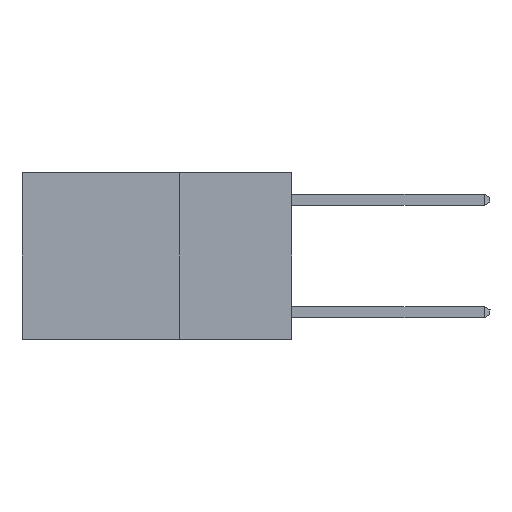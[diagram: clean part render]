
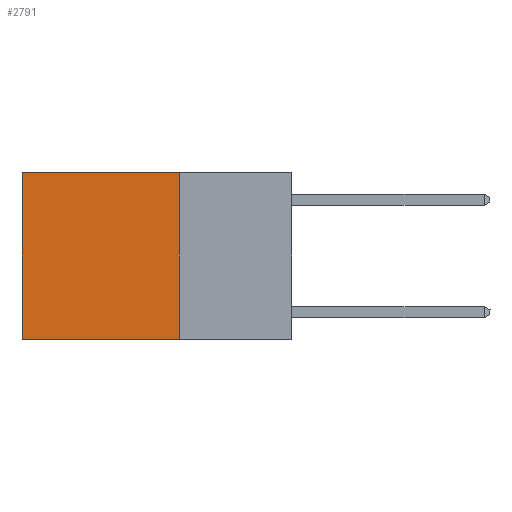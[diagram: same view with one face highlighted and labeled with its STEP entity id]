
A CAD part, left-side view. The second image highlights one B-rep face of the part: STEP entity #2791.
In plain terms, the highlighted planar face has unit normal (-1, 0, 0).
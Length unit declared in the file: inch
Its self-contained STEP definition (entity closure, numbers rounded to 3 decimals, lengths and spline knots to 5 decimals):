
#106 = CARTESIAN_POINT ( 'NONE',  ( 0.2625, 0.6, -0.37 ) ) ;
#130 = ORIENTED_EDGE ( 'NONE', *, *, #4910, .T. ) ;
#237 = ORIENTED_EDGE ( 'NONE', *, *, #2673, .T. ) ;
#852 = ORIENTED_EDGE ( 'NONE', *, *, #1747, .F. ) ;
#915 = ORIENTED_EDGE ( 'NONE', *, *, #6691, .F. ) ;
#1747 = EDGE_CURVE ( 'NONE', #3632, #5428, #7974, .T. ) ;
#1890 = LINE ( 'NONE', #3417, #10299 ) ;
#2107 = DIRECTION ( 'NONE',  ( 0., 1., 0. ) ) ;
#2298 = CARTESIAN_POINT ( 'NONE',  ( 0.2625, 0.25, 0. ) ) ;
#2512 = CARTESIAN_POINT ( 'NONE',  ( 0.2625, 0.6, 0. ) ) ;
#2673 = EDGE_CURVE ( 'NONE', #3632, #8798, #5055, .T. ) ;
#2791 = ADVANCED_FACE ( 'NONE', ( #6189 ), #8386, .F. ) ;
#2939 = VERTEX_POINT ( 'NONE', #106 ) ;
#2976 = CARTESIAN_POINT ( 'NONE',  ( 0.2625, 0.25, 0. ) ) ;
#3417 = CARTESIAN_POINT ( 'NONE',  ( 0.2625, 0.6, 0. ) ) ;
#3632 = VERTEX_POINT ( 'NONE', #2976 ) ;
#4337 = CARTESIAN_POINT ( 'NONE',  ( 0.2625, 0.25, 0. ) ) ;
#4779 = DIRECTION ( 'NONE',  ( 0., 0., -1. ) ) ;
#4910 = EDGE_CURVE ( 'NONE', #8798, #2939, #1890, .T. ) ;
#5055 = LINE ( 'NONE', #9016, #9066 ) ;
#5203 = DIRECTION ( 'NONE',  ( 0., 0., -1. ) ) ;
#5428 = VERTEX_POINT ( 'NONE', #7160 ) ;
#6189 = FACE_OUTER_BOUND ( 'NONE', #7083, .T. ) ;
#6691 = EDGE_CURVE ( 'NONE', #5428, #2939, #7344, .T. ) ;
#7083 = EDGE_LOOP ( 'NONE', ( #130, #915, #852, #237 ) ) ;
#7160 = CARTESIAN_POINT ( 'NONE',  ( 0.2625, 0.25, -0.37 ) ) ;
#7344 = LINE ( 'NONE', #7818, #9224 ) ;
#7622 = AXIS2_PLACEMENT_3D ( 'NONE', #4337, #9985, #5203 ) ;
#7818 = CARTESIAN_POINT ( 'NONE',  ( 0.2625, 0.25, -0.37 ) ) ;
#7974 = LINE ( 'NONE', #2298, #9844 ) ;
#8386 = PLANE ( 'NONE',  #7622 ) ;
#8798 = VERTEX_POINT ( 'NONE', #2512 ) ;
#9016 = CARTESIAN_POINT ( 'NONE',  ( 0.2625, 0.25, 0. ) ) ;
#9066 = VECTOR ( 'NONE', #9809, 39.37008 ) ;
#9224 = VECTOR ( 'NONE', #2107, 39.37008 ) ;
#9809 = DIRECTION ( 'NONE',  ( 0., 1., 0. ) ) ;
#9844 = VECTOR ( 'NONE', #4779, 39.37008 ) ;
#9985 = DIRECTION ( 'NONE',  ( 1., 0., 0. ) ) ;
#10299 = VECTOR ( 'NONE', #10686, 39.37008 ) ;
#10686 = DIRECTION ( 'NONE',  ( 0., 0., -1. ) ) ;
